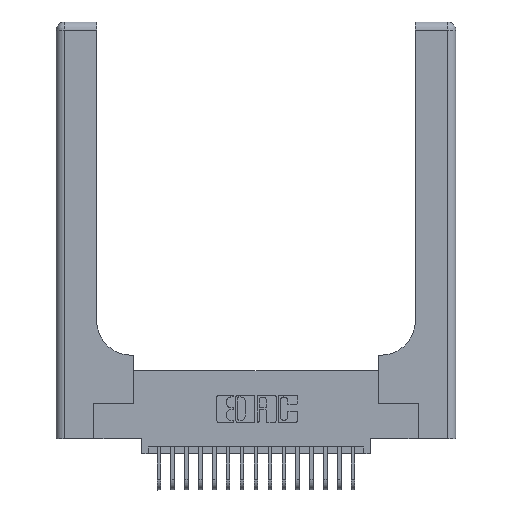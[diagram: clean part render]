
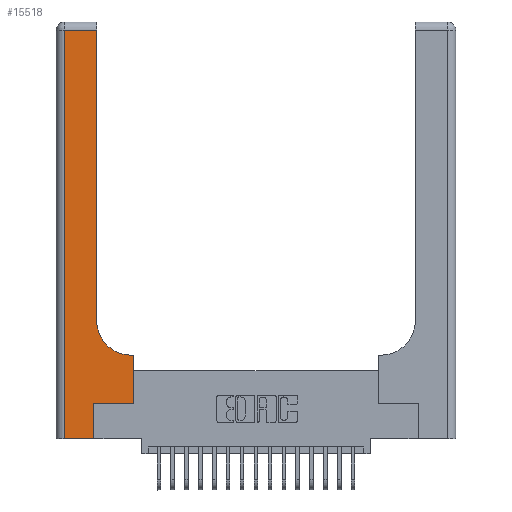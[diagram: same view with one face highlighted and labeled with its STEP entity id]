
A CAD part, top view. The second image highlights one B-rep face of the part: STEP entity #15518.
In plain terms, the highlighted planar face has unit normal (0, 0, 1).
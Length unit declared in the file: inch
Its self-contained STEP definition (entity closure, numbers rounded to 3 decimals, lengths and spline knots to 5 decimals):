
#356 = EDGE_LOOP ( 'NONE', ( #14961, #7590, #5876, #7623, #10955, #13204, #15792, #13483, #13509 ) ) ;
#466 = LINE ( 'NONE', #20062, #16693 ) ;
#593 = CARTESIAN_POINT ( 'NONE',  ( 0.269, 0.25, 0.37 ) ) ;
#873 = DIRECTION ( 'NONE',  ( 0., 1., 0. ) ) ;
#1505 = CARTESIAN_POINT ( 'NONE',  ( 0.269, 0., 0.37 ) ) ;
#1517 = EDGE_CURVE ( 'NONE', #5635, #10099, #2047, .T. ) ;
#1630 = CARTESIAN_POINT ( 'NONE',  ( 0.06, 0., 0.37 ) ) ;
#1670 = VERTEX_POINT ( 'NONE', #2934 ) ;
#1766 = LINE ( 'NONE', #6137, #17484 ) ;
#2047 = LINE ( 'NONE', #19680, #17775 ) ;
#2260 = EDGE_CURVE ( 'NONE', #4903, #11952, #1766, .T. ) ;
#2452 = EDGE_CURVE ( 'NONE', #1670, #4903, #5662, .T. ) ;
#2811 = CARTESIAN_POINT ( 'NONE',  ( 0.5585, 0.6, 0.37 ) ) ;
#2934 = CARTESIAN_POINT ( 'NONE',  ( 0.06, 2.94, 0.37 ) ) ;
#3474 = EDGE_CURVE ( 'NONE', #18059, #13349, #466, .T. ) ;
#4301 = PLANE ( 'NONE',  #12569 ) ;
#4376 = CARTESIAN_POINT ( 'NONE',  ( 0., 2.94, 0.37 ) ) ;
#4903 = VERTEX_POINT ( 'NONE', #1630 ) ;
#5635 = VERTEX_POINT ( 'NONE', #19299 ) ;
#5662 = LINE ( 'NONE', #17609, #14574 ) ;
#5850 = DIRECTION ( 'NONE',  ( 0., 0., -1. ) ) ;
#5876 = ORIENTED_EDGE ( 'NONE', *, *, #2452, .T. ) ;
#6027 = DIRECTION ( 'NONE',  ( 0., 1., 0. ) ) ;
#6137 = CARTESIAN_POINT ( 'NONE',  ( 0., 0., 0.37 ) ) ;
#6139 = EDGE_CURVE ( 'NONE', #10245, #18059, #13208, .T. ) ;
#6803 = CARTESIAN_POINT ( 'NONE',  ( 0.5415, 0.85, 0.37 ) ) ;
#7531 = DIRECTION ( 'NONE',  ( -1., 0., 0. ) ) ;
#7590 = ORIENTED_EDGE ( 'NONE', *, *, #13923, .T. ) ;
#7623 = ORIENTED_EDGE ( 'NONE', *, *, #2260, .T. ) ;
#7910 = CARTESIAN_POINT ( 'NONE',  ( 0.2915, 2.94, 0.37 ) ) ;
#8219 = DIRECTION ( 'NONE',  ( 0., -1., 0. ) ) ;
#8394 = DIRECTION ( 'NONE',  ( 1., 0., 0. ) ) ;
#8509 = EDGE_CURVE ( 'NONE', #20149, #5635, #15465, .T. ) ;
#8595 = DIRECTION ( 'NONE',  ( -1., 0., 0. ) ) ;
#8631 = EDGE_CURVE ( 'NONE', #11952, #20149, #14495, .T. ) ;
#8805 = VECTOR ( 'NONE', #10938, 39.37008 ) ;
#9432 = VECTOR ( 'NONE', #7531, 39.37008 ) ;
#9587 = CARTESIAN_POINT ( 'NONE',  ( 0.269, 0., 0.37 ) ) ;
#10099 = VERTEX_POINT ( 'NONE', #2811 ) ;
#10245 = VERTEX_POINT ( 'NONE', #14316 ) ;
#10850 = DIRECTION ( 'NONE',  ( 1., 0., 0. ) ) ;
#10938 = DIRECTION ( 'NONE',  ( 0., 1., 0. ) ) ;
#10955 = ORIENTED_EDGE ( 'NONE', *, *, #8631, .T. ) ;
#11300 = VECTOR ( 'NONE', #12236, 39.37008 ) ;
#11952 = VERTEX_POINT ( 'NONE', #1505 ) ;
#12236 = DIRECTION ( 'NONE',  ( 1., 0., 0. ) ) ;
#12569 = AXIS2_PLACEMENT_3D ( 'NONE', #13743, #5850, #16856 ) ;
#13204 = ORIENTED_EDGE ( 'NONE', *, *, #8509, .T. ) ;
#13208 = CIRCLE ( 'NONE', #15430, 0.25 ) ;
#13349 = VERTEX_POINT ( 'NONE', #7910 ) ;
#13483 = ORIENTED_EDGE ( 'NONE', *, *, #13645, .T. ) ;
#13509 = ORIENTED_EDGE ( 'NONE', *, *, #6139, .T. ) ;
#13619 = FACE_OUTER_BOUND ( 'NONE', #356, .T. ) ;
#13645 = EDGE_CURVE ( 'NONE', #10099, #10245, #18495, .T. ) ;
#13743 = CARTESIAN_POINT ( 'NONE',  ( 0., 3., 0.37 ) ) ;
#13923 = EDGE_CURVE ( 'NONE', #13349, #1670, #14646, .T. ) ;
#14316 = CARTESIAN_POINT ( 'NONE',  ( 0.5415, 0.6, 0.37 ) ) ;
#14495 = LINE ( 'NONE', #9587, #8805 ) ;
#14574 = VECTOR ( 'NONE', #8219, 39.37008 ) ;
#14646 = LINE ( 'NONE', #4376, #9432 ) ;
#14895 = VECTOR ( 'NONE', #8595, 39.37008 ) ;
#14961 = ORIENTED_EDGE ( 'NONE', *, *, #3474, .T. ) ;
#15265 = CARTESIAN_POINT ( 'NONE',  ( 0.2915, 0.85, 0.37 ) ) ;
#15430 = AXIS2_PLACEMENT_3D ( 'NONE', #6803, #17800, #8394 ) ;
#15465 = LINE ( 'NONE', #19988, #11300 ) ;
#15518 = ADVANCED_FACE ( 'NONE', ( #13619 ), #4301, .F. ) ;
#15792 = ORIENTED_EDGE ( 'NONE', *, *, #1517, .T. ) ;
#16693 = VECTOR ( 'NONE', #6027, 39.37008 ) ;
#16856 = DIRECTION ( 'NONE',  ( -1., 0., 0. ) ) ;
#17484 = VECTOR ( 'NONE', #10850, 39.37008 ) ;
#17609 = CARTESIAN_POINT ( 'NONE',  ( 0.06, 3., 0.37 ) ) ;
#17775 = VECTOR ( 'NONE', #873, 39.37008 ) ;
#17800 = DIRECTION ( 'NONE',  ( 0., 0., -1. ) ) ;
#17980 = CARTESIAN_POINT ( 'NONE',  ( 0.2915, 0.6, 0.37 ) ) ;
#18059 = VERTEX_POINT ( 'NONE', #15265 ) ;
#18495 = LINE ( 'NONE', #17980, #14895 ) ;
#19299 = CARTESIAN_POINT ( 'NONE',  ( 0.5585, 0.25, 0.37 ) ) ;
#19680 = CARTESIAN_POINT ( 'NONE',  ( 0.5585, 0.25, 0.37 ) ) ;
#19988 = CARTESIAN_POINT ( 'NONE',  ( 0.269, 0.25, 0.37 ) ) ;
#20062 = CARTESIAN_POINT ( 'NONE',  ( 0.2915, 3., 0.37 ) ) ;
#20149 = VERTEX_POINT ( 'NONE', #593 ) ;
